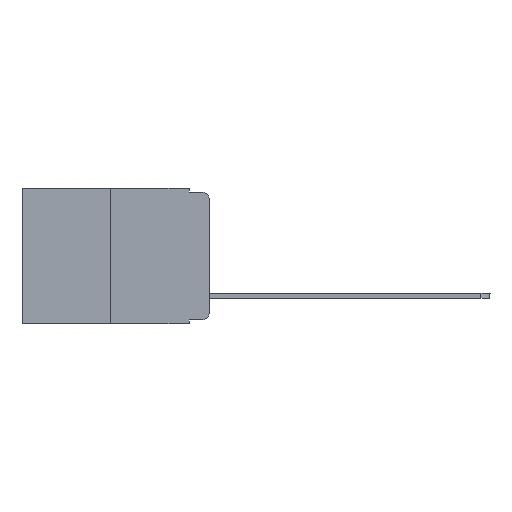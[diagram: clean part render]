
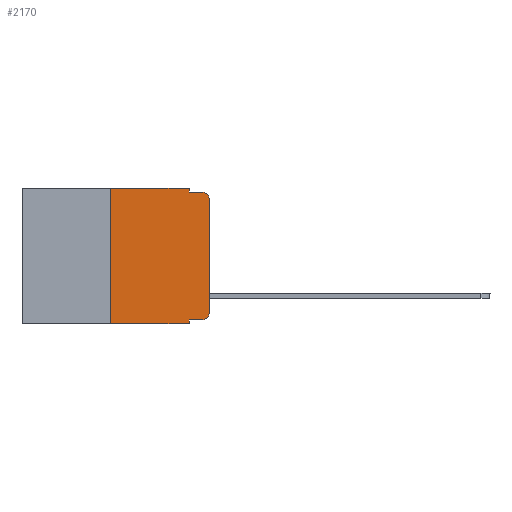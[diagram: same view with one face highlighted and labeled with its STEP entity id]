
A CAD part, left-side view. The second image highlights one B-rep face of the part: STEP entity #2170.
In plain terms, the highlighted planar face has unit normal (-1, 0, 0).
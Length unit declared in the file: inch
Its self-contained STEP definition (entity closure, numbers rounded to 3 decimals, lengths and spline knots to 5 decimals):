
#348 = CARTESIAN_POINT ( 'NONE',  ( 0., 0., -0.03 ) ) ;
#641 = ORIENTED_EDGE ( 'NONE', *, *, #17148, .T. ) ;
#814 = VERTEX_POINT ( 'NONE', #9425 ) ;
#1399 = LINE ( 'NONE', #11738, #18393 ) ;
#1450 = EDGE_CURVE ( 'NONE', #3868, #9305, #10042, .T. ) ;
#1753 = DIRECTION ( 'NONE',  ( -1., 0., 0. ) ) ;
#1999 = VERTEX_POINT ( 'NONE', #2206 ) ;
#2170 = ADVANCED_FACE ( 'NONE', ( #12547 ), #17494, .F. ) ;
#2206 = CARTESIAN_POINT ( 'NONE',  ( 0., 0.051, -0.343 ) ) ;
#2794 = AXIS2_PLACEMENT_3D ( 'NONE', #15676, #20510, #20618 ) ;
#2833 = CARTESIAN_POINT ( 'NONE',  ( 0., 0.473, -0.343 ) ) ;
#2859 = DIRECTION ( 'NONE',  ( 0., 0., 1. ) ) ;
#2882 = DIRECTION ( 'NONE',  ( 0., 0., -1. ) ) ;
#3067 = EDGE_CURVE ( 'NONE', #3868, #1999, #17627, .T. ) ;
#3185 = CARTESIAN_POINT ( 'NONE',  ( 0., 0.25, 0. ) ) ;
#3291 = DIRECTION ( 'NONE',  ( 0., -1., 0. ) ) ;
#3868 = VERTEX_POINT ( 'NONE', #5796 ) ;
#4533 = CARTESIAN_POINT ( 'NONE',  ( 0., 0.051, 0. ) ) ;
#4797 = VECTOR ( 'NONE', #3291, 39.37008 ) ;
#5243 = CIRCLE ( 'NONE', #2794, 0.02 ) ;
#5289 = EDGE_CURVE ( 'NONE', #12340, #814, #6576, .T. ) ;
#5796 = CARTESIAN_POINT ( 'NONE',  ( 0., 0.051, -0.333 ) ) ;
#5909 = EDGE_CURVE ( 'NONE', #20663, #18139, #9181, .T. ) ;
#5979 = DIRECTION ( 'NONE',  ( 0., -1., 0. ) ) ;
#6254 = LINE ( 'NONE', #3185, #15918 ) ;
#6576 = LINE ( 'NONE', #11641, #4797 ) ;
#6811 = ORIENTED_EDGE ( 'NONE', *, *, #18468, .T. ) ;
#7213 = AXIS2_PLACEMENT_3D ( 'NONE', #9121, #7463, #17596 ) ;
#7463 = DIRECTION ( 'NONE',  ( 1., 0., 0. ) ) ;
#7900 = VERTEX_POINT ( 'NONE', #348 ) ;
#7942 = ORIENTED_EDGE ( 'NONE', *, *, #17546, .F. ) ;
#8630 = CARTESIAN_POINT ( 'NONE',  ( 0., 0.02, -0.333 ) ) ;
#9121 = CARTESIAN_POINT ( 'NONE',  ( 0., 0.473, 0. ) ) ;
#9181 = LINE ( 'NONE', #19307, #16174 ) ;
#9305 = VERTEX_POINT ( 'NONE', #8630 ) ;
#9425 = CARTESIAN_POINT ( 'NONE',  ( 0., 0.02, -0.01 ) ) ;
#9810 = ORIENTED_EDGE ( 'NONE', *, *, #5909, .F. ) ;
#10042 = LINE ( 'NONE', #21719, #18098 ) ;
#10132 = CARTESIAN_POINT ( 'NONE',  ( 0., 0.25, -0.343 ) ) ;
#10133 = EDGE_LOOP ( 'NONE', ( #641, #6811, #15042, #7942, #9810, #17273, #18881, #16480, #13386, #15230 ) ) ;
#10548 = VECTOR ( 'NONE', #12955, 39.37008 ) ;
#10771 = VECTOR ( 'NONE', #2882, 39.37008 ) ;
#11218 = LINE ( 'NONE', #17931, #19445 ) ;
#11641 = CARTESIAN_POINT ( 'NONE',  ( 0., 0.051, -0.01 ) ) ;
#11738 = CARTESIAN_POINT ( 'NONE',  ( 0., 0.051, 0. ) ) ;
#11756 = CIRCLE ( 'NONE', #17733, 0.02 ) ;
#11780 = VERTEX_POINT ( 'NONE', #17442 ) ;
#12340 = VERTEX_POINT ( 'NONE', #14759 ) ;
#12547 = FACE_OUTER_BOUND ( 'NONE', #10133, .T. ) ;
#12879 = DIRECTION ( 'NONE',  ( 0., 0., 1. ) ) ;
#12955 = DIRECTION ( 'NONE',  ( 0., -1., 0. ) ) ;
#13386 = ORIENTED_EDGE ( 'NONE', *, *, #1450, .T. ) ;
#13848 = DIRECTION ( 'NONE',  ( 0., 0., -1. ) ) ;
#14759 = CARTESIAN_POINT ( 'NONE',  ( 0., 0.051, -0.01 ) ) ;
#15042 = ORIENTED_EDGE ( 'NONE', *, *, #5289, .F. ) ;
#15100 = DIRECTION ( 'NONE',  ( 0., -1., 0. ) ) ;
#15230 = ORIENTED_EDGE ( 'NONE', *, *, #19546, .T. ) ;
#15676 = CARTESIAN_POINT ( 'NONE',  ( 0., 0.02, -0.313 ) ) ;
#15918 = VECTOR ( 'NONE', #12879, 39.37008 ) ;
#16174 = VECTOR ( 'NONE', #5979, 39.37008 ) ;
#16480 = ORIENTED_EDGE ( 'NONE', *, *, #3067, .F. ) ;
#17048 = CARTESIAN_POINT ( 'NONE',  ( 0., 0.02, -0.03 ) ) ;
#17119 = EDGE_CURVE ( 'NONE', #19750, #20663, #6254, .T. ) ;
#17148 = EDGE_CURVE ( 'NONE', #11780, #7900, #11218, .T. ) ;
#17273 = ORIENTED_EDGE ( 'NONE', *, *, #17119, .F. ) ;
#17442 = CARTESIAN_POINT ( 'NONE',  ( 0., 0., -0.313 ) ) ;
#17494 = PLANE ( 'NONE',  #7213 ) ;
#17546 = EDGE_CURVE ( 'NONE', #18139, #12340, #1399, .T. ) ;
#17596 = DIRECTION ( 'NONE',  ( 0., 0., -1. ) ) ;
#17627 = LINE ( 'NONE', #4533, #10771 ) ;
#17733 = AXIS2_PLACEMENT_3D ( 'NONE', #17048, #1753, #13848 ) ;
#17839 = CARTESIAN_POINT ( 'NONE',  ( 0., 0.051, 0. ) ) ;
#17931 = CARTESIAN_POINT ( 'NONE',  ( 0., 0., 0. ) ) ;
#18098 = VECTOR ( 'NONE', #15100, 39.37008 ) ;
#18139 = VERTEX_POINT ( 'NONE', #17839 ) ;
#18332 = DIRECTION ( 'NONE',  ( 0., 0., -1. ) ) ;
#18393 = VECTOR ( 'NONE', #18332, 39.37008 ) ;
#18468 = EDGE_CURVE ( 'NONE', #7900, #814, #11756, .T. ) ;
#18813 = EDGE_CURVE ( 'NONE', #19750, #1999, #21653, .T. ) ;
#18881 = ORIENTED_EDGE ( 'NONE', *, *, #18813, .T. ) ;
#19005 = CARTESIAN_POINT ( 'NONE',  ( 0., 0.25, 0. ) ) ;
#19307 = CARTESIAN_POINT ( 'NONE',  ( 0., 0.473, 0. ) ) ;
#19445 = VECTOR ( 'NONE', #2859, 39.37008 ) ;
#19546 = EDGE_CURVE ( 'NONE', #9305, #11780, #5243, .T. ) ;
#19750 = VERTEX_POINT ( 'NONE', #10132 ) ;
#20510 = DIRECTION ( 'NONE',  ( -1., 0., 0. ) ) ;
#20618 = DIRECTION ( 'NONE',  ( 0., 0., -1. ) ) ;
#20663 = VERTEX_POINT ( 'NONE', #19005 ) ;
#21653 = LINE ( 'NONE', #2833, #10548 ) ;
#21719 = CARTESIAN_POINT ( 'NONE',  ( 0., 0.051, -0.333 ) ) ;
